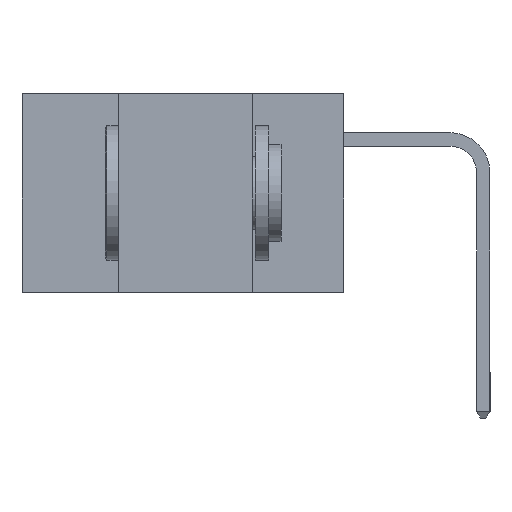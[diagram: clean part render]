
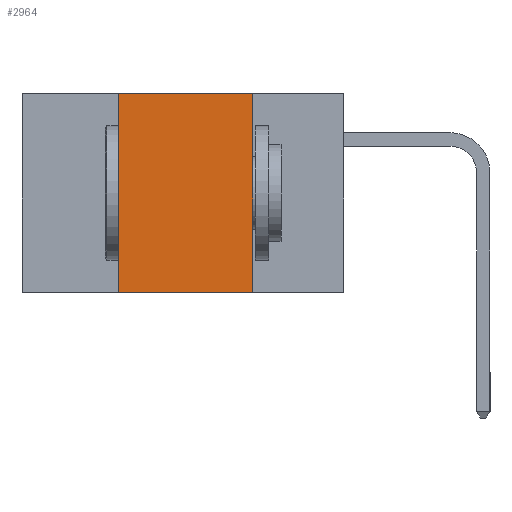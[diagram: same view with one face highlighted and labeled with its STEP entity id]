
A CAD part, left-side view. The second image highlights one B-rep face of the part: STEP entity #2964.
In plain terms, the highlighted planar face has unit normal (-1, 0, 0).
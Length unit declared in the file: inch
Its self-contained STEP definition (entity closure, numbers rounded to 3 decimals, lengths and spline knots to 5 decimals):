
#162 = VERTEX_POINT ( 'NONE', #2715 ) ;
#166 = VERTEX_POINT ( 'NONE', #8051 ) ;
#678 = DIRECTION ( 'NONE',  ( 1., 0., 0. ) ) ;
#1470 = FACE_OUTER_BOUND ( 'NONE', #2109, .T. ) ;
#1598 = CARTESIAN_POINT ( 'NONE',  ( 0., 0.6, 0. ) ) ;
#1711 = CARTESIAN_POINT ( 'NONE',  ( 0., 0.42, 0. ) ) ;
#2075 = EDGE_CURVE ( 'NONE', #11707, #166, #6396, .T. ) ;
#2109 = EDGE_LOOP ( 'NONE', ( #6323, #3905, #10824, #10814 ) ) ;
#2282 = EDGE_CURVE ( 'NONE', #166, #162, #9318, .T. ) ;
#2358 = DIRECTION ( 'NONE',  ( 0., 0., 1. ) ) ;
#2564 = AXIS2_PLACEMENT_3D ( 'NONE', #1598, #678, #4453 ) ;
#2682 = CARTESIAN_POINT ( 'NONE',  ( 0., 0.17, -0.37 ) ) ;
#2715 = CARTESIAN_POINT ( 'NONE',  ( 0., 0.17, -0.37 ) ) ;
#2927 = VECTOR ( 'NONE', #10206, 39.37008 ) ;
#2964 = ADVANCED_FACE ( 'NONE', ( #1470 ), #9973, .F. ) ;
#3622 = DIRECTION ( 'NONE',  ( 0., -1., 0. ) ) ;
#3679 = LINE ( 'NONE', #10054, #7870 ) ;
#3905 = ORIENTED_EDGE ( 'NONE', *, *, #2075, .F. ) ;
#4252 = EDGE_CURVE ( 'NONE', #10155, #162, #3679, .T. ) ;
#4391 = VECTOR ( 'NONE', #2358, 39.37008 ) ;
#4453 = DIRECTION ( 'NONE',  ( 0., 0., -1. ) ) ;
#4905 = VECTOR ( 'NONE', #6414, 39.37008 ) ;
#5919 = EDGE_CURVE ( 'NONE', #10155, #11707, #9131, .T. ) ;
#6323 = ORIENTED_EDGE ( 'NONE', *, *, #2282, .F. ) ;
#6396 = LINE ( 'NONE', #7378, #2927 ) ;
#6414 = DIRECTION ( 'NONE',  ( 0., 0., -1. ) ) ;
#7378 = CARTESIAN_POINT ( 'NONE',  ( 0., 0.6, 0. ) ) ;
#7870 = VECTOR ( 'NONE', #3622, 39.37008 ) ;
#8051 = CARTESIAN_POINT ( 'NONE',  ( 0., 0.17, 0. ) ) ;
#8131 = CARTESIAN_POINT ( 'NONE',  ( 0., 0.42, -0.37 ) ) ;
#9131 = LINE ( 'NONE', #8131, #4391 ) ;
#9318 = LINE ( 'NONE', #2682, #4905 ) ;
#9578 = CARTESIAN_POINT ( 'NONE',  ( 0., 0.42, -0.37 ) ) ;
#9973 = PLANE ( 'NONE',  #2564 ) ;
#10054 = CARTESIAN_POINT ( 'NONE',  ( 0., 0.6, -0.37 ) ) ;
#10155 = VERTEX_POINT ( 'NONE', #9578 ) ;
#10206 = DIRECTION ( 'NONE',  ( 0., -1., 0. ) ) ;
#10814 = ORIENTED_EDGE ( 'NONE', *, *, #4252, .T. ) ;
#10824 = ORIENTED_EDGE ( 'NONE', *, *, #5919, .F. ) ;
#11707 = VERTEX_POINT ( 'NONE', #1711 ) ;
